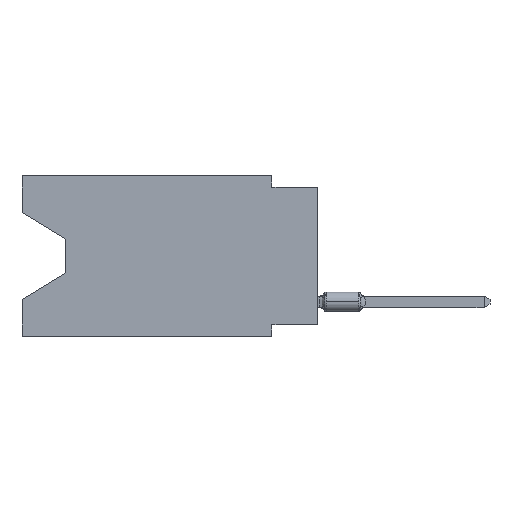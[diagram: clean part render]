
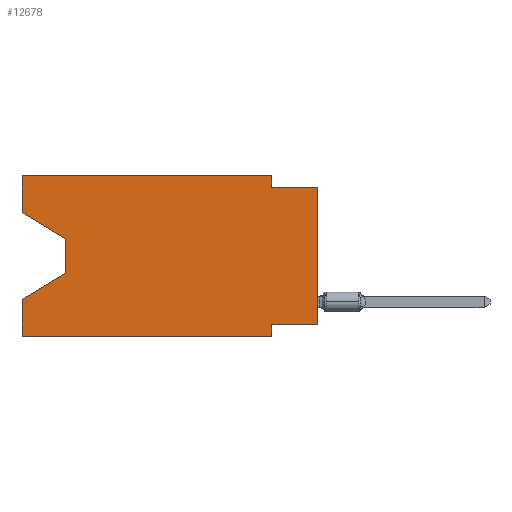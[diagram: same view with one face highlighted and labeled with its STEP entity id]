
A CAD part, left-side view. The second image highlights one B-rep face of the part: STEP entity #12678.
In plain terms, the highlighted planar face has unit normal (-1, 0, 0).
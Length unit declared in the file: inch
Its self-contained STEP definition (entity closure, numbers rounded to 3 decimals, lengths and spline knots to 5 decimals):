
#699 = ORIENTED_EDGE ( 'NONE', *, *, #8091, .T. ) ;
#731 = VERTEX_POINT ( 'NONE', #2712 ) ;
#733 = EDGE_CURVE ( 'NONE', #13369, #731, #6883, .T. ) ;
#850 = CARTESIAN_POINT ( 'NONE',  ( 0., 0.1, 0. ) ) ;
#881 = ORIENTED_EDGE ( 'NONE', *, *, #10073, .T. ) ;
#928 = LINE ( 'NONE', #5152, #3778 ) ;
#999 = CARTESIAN_POINT ( 'NONE',  ( 0., 0.1, -0.35 ) ) ;
#1003 = ORIENTED_EDGE ( 'NONE', *, *, #8249, .T. ) ;
#1096 = LINE ( 'NONE', #7231, #4834 ) ;
#1467 = EDGE_CURVE ( 'NONE', #11748, #10804, #11449, .T. ) ;
#1557 = CARTESIAN_POINT ( 'NONE',  ( 0., 0.1, -0.35 ) ) ;
#2444 = CARTESIAN_POINT ( 'NONE',  ( 0., 0., -0.025 ) ) ;
#2496 = VECTOR ( 'NONE', #2603, 39.37008 ) ;
#2547 = ORIENTED_EDGE ( 'NONE', *, *, #5865, .F. ) ;
#2603 = DIRECTION ( 'NONE',  ( 0., 1., 0. ) ) ;
#2709 = VECTOR ( 'NONE', #3960, 39.37008 ) ;
#2712 = CARTESIAN_POINT ( 'NONE',  ( 0., 0., -0.025 ) ) ;
#2825 = EDGE_CURVE ( 'NONE', #8365, #3685, #10812, .T. ) ;
#2925 = EDGE_LOOP ( 'NONE', ( #1003, #699, #8816, #5090, #13340, #10659, #7542, #881, #12343, #6385, #2547, #12736 ) ) ;
#2971 = DIRECTION ( 'NONE',  ( 0., 0., -1. ) ) ;
#3249 = DIRECTION ( 'NONE',  ( 0., 0., -1. ) ) ;
#3513 = CARTESIAN_POINT ( 'NONE',  ( 0., 0.1, -0.325 ) ) ;
#3685 = VERTEX_POINT ( 'NONE', #3513 ) ;
#3778 = VECTOR ( 'NONE', #13415, 39.37008 ) ;
#3960 = DIRECTION ( 'NONE',  ( 0., 0., -1. ) ) ;
#3964 = VERTEX_POINT ( 'NONE', #12717 ) ;
#4301 = EDGE_CURVE ( 'NONE', #7107, #3964, #1096, .T. ) ;
#4528 = VERTEX_POINT ( 'NONE', #11892 ) ;
#4702 = DIRECTION ( 'NONE',  ( 0., -0.855, -0.519 ) ) ;
#4834 = VECTOR ( 'NONE', #8465, 39.37008 ) ;
#5090 = ORIENTED_EDGE ( 'NONE', *, *, #7260, .F. ) ;
#5152 = CARTESIAN_POINT ( 'NONE',  ( 0., 0.645, 0. ) ) ;
#5156 = AXIS2_PLACEMENT_3D ( 'NONE', #9793, #8833, #7598 ) ;
#5200 = EDGE_CURVE ( 'NONE', #12829, #13369, #8434, .T. ) ;
#5478 = FACE_OUTER_BOUND ( 'NONE', #2925, .T. ) ;
#5513 = VECTOR ( 'NONE', #7658, 39.37008 ) ;
#5555 = CARTESIAN_POINT ( 'NONE',  ( 0., 0.645, -0.35 ) ) ;
#5640 = LINE ( 'NONE', #7671, #9940 ) ;
#5862 = CARTESIAN_POINT ( 'NONE',  ( 0., 0.1, -0.025 ) ) ;
#5865 = EDGE_CURVE ( 'NONE', #3964, #12829, #11804, .T. ) ;
#5913 = VERTEX_POINT ( 'NONE', #8784 ) ;
#5920 = CARTESIAN_POINT ( 'NONE',  ( 0., 0., -0.325 ) ) ;
#6066 = CARTESIAN_POINT ( 'NONE',  ( 0., 0.55, -0.212 ) ) ;
#6214 = VERTEX_POINT ( 'NONE', #9655 ) ;
#6385 = ORIENTED_EDGE ( 'NONE', *, *, #5200, .F. ) ;
#6600 = DIRECTION ( 'NONE',  ( 0., -1., 0. ) ) ;
#6692 = LINE ( 'NONE', #8802, #11662 ) ;
#6883 = LINE ( 'NONE', #2444, #11492 ) ;
#6968 = LINE ( 'NONE', #12435, #2709 ) ;
#7107 = VERTEX_POINT ( 'NONE', #11114 ) ;
#7231 = CARTESIAN_POINT ( 'NONE',  ( 0., 0.645, 0. ) ) ;
#7260 = EDGE_CURVE ( 'NONE', #11748, #6214, #928, .T. ) ;
#7301 = EDGE_CURVE ( 'NONE', #3685, #10804, #9327, .T. ) ;
#7542 = ORIENTED_EDGE ( 'NONE', *, *, #2825, .F. ) ;
#7598 = DIRECTION ( 'NONE',  ( 0., 0., -1. ) ) ;
#7658 = DIRECTION ( 'NONE',  ( 0., -1., 0. ) ) ;
#7671 = CARTESIAN_POINT ( 'NONE',  ( 0., 0., 0. ) ) ;
#8091 = EDGE_CURVE ( 'NONE', #4528, #5913, #6968, .T. ) ;
#8107 = VECTOR ( 'NONE', #6600, 39.37008 ) ;
#8249 = EDGE_CURVE ( 'NONE', #7107, #4528, #6692, .T. ) ;
#8365 = VERTEX_POINT ( 'NONE', #5920 ) ;
#8434 = LINE ( 'NONE', #13486, #12495 ) ;
#8465 = DIRECTION ( 'NONE',  ( 0., 0., 1. ) ) ;
#8784 = CARTESIAN_POINT ( 'NONE',  ( 0., 0.55, -0.212 ) ) ;
#8802 = CARTESIAN_POINT ( 'NONE',  ( 0., 0.645, -0.08025 ) ) ;
#8816 = ORIENTED_EDGE ( 'NONE', *, *, #13500, .T. ) ;
#8833 = DIRECTION ( 'NONE',  ( 1., 0., 0. ) ) ;
#8997 = DIRECTION ( 'NONE',  ( 0., -1., 0. ) ) ;
#9327 = LINE ( 'NONE', #999, #13375 ) ;
#9345 = DIRECTION ( 'NONE',  ( 0., 0.855, -0.519 ) ) ;
#9655 = CARTESIAN_POINT ( 'NONE',  ( 0., 0.645, -0.26975 ) ) ;
#9793 = CARTESIAN_POINT ( 'NONE',  ( 0., 0.645, 0. ) ) ;
#9940 = VECTOR ( 'NONE', #10906, 39.37008 ) ;
#10073 = EDGE_CURVE ( 'NONE', #8365, #731, #5640, .T. ) ;
#10659 = ORIENTED_EDGE ( 'NONE', *, *, #7301, .F. ) ;
#10804 = VERTEX_POINT ( 'NONE', #1557 ) ;
#10812 = LINE ( 'NONE', #11834, #2496 ) ;
#10863 = VECTOR ( 'NONE', #9345, 39.37008 ) ;
#10906 = DIRECTION ( 'NONE',  ( 0., 0., 1. ) ) ;
#11114 = CARTESIAN_POINT ( 'NONE',  ( 0., 0.645, -0.08025 ) ) ;
#11449 = LINE ( 'NONE', #5555, #5513 ) ;
#11492 = VECTOR ( 'NONE', #8997, 39.37008 ) ;
#11662 = VECTOR ( 'NONE', #4702, 39.37008 ) ;
#11748 = VERTEX_POINT ( 'NONE', #12999 ) ;
#11804 = LINE ( 'NONE', #12823, #8107 ) ;
#11834 = CARTESIAN_POINT ( 'NONE',  ( 0., 0., -0.325 ) ) ;
#11892 = CARTESIAN_POINT ( 'NONE',  ( 0., 0.55, -0.138 ) ) ;
#12343 = ORIENTED_EDGE ( 'NONE', *, *, #733, .F. ) ;
#12435 = CARTESIAN_POINT ( 'NONE',  ( 0., 0.55, -0.138 ) ) ;
#12495 = VECTOR ( 'NONE', #3249, 39.37008 ) ;
#12678 = ADVANCED_FACE ( 'NONE', ( #5478 ), #12867, .F. ) ;
#12717 = CARTESIAN_POINT ( 'NONE',  ( 0., 0.645, 0. ) ) ;
#12736 = ORIENTED_EDGE ( 'NONE', *, *, #4301, .F. ) ;
#12823 = CARTESIAN_POINT ( 'NONE',  ( 0., 0.645, 0. ) ) ;
#12829 = VERTEX_POINT ( 'NONE', #850 ) ;
#12867 = PLANE ( 'NONE',  #5156 ) ;
#12999 = CARTESIAN_POINT ( 'NONE',  ( 0., 0.645, -0.35 ) ) ;
#13340 = ORIENTED_EDGE ( 'NONE', *, *, #1467, .T. ) ;
#13368 = LINE ( 'NONE', #6066, #10863 ) ;
#13369 = VERTEX_POINT ( 'NONE', #5862 ) ;
#13375 = VECTOR ( 'NONE', #2971, 39.37008 ) ;
#13415 = DIRECTION ( 'NONE',  ( 0., 0., 1. ) ) ;
#13486 = CARTESIAN_POINT ( 'NONE',  ( 0., 0.1, 0. ) ) ;
#13500 = EDGE_CURVE ( 'NONE', #5913, #6214, #13368, .T. ) ;
